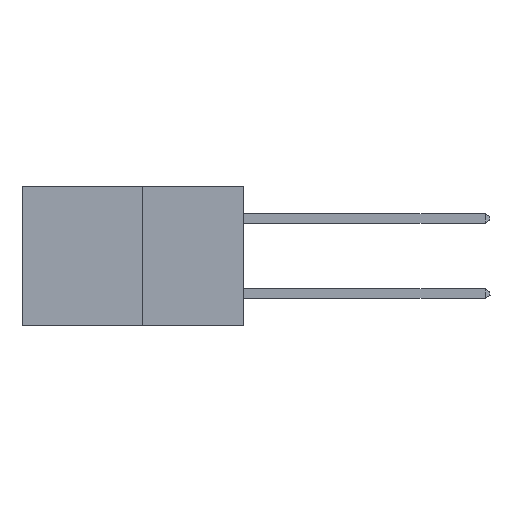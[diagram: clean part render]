
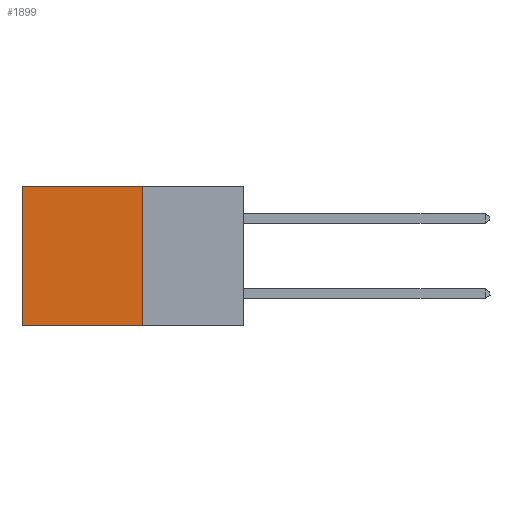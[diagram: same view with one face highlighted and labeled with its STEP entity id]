
A CAD part, left-side view. The second image highlights one B-rep face of the part: STEP entity #1899.
In plain terms, the highlighted planar face has unit normal (-1, 0, 0).
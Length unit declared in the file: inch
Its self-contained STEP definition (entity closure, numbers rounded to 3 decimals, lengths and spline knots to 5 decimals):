
#274 = EDGE_CURVE ( 'NONE', #8923, #3825, #8251, .T. ) ;
#282 = LINE ( 'NONE', #6244, #6192 ) ;
#631 = AXIS2_PLACEMENT_3D ( 'NONE', #7291, #9025, #3085 ) ;
#766 = EDGE_CURVE ( 'NONE', #3419, #8923, #282, .T. ) ;
#1061 = LINE ( 'NONE', #7419, #8402 ) ;
#1638 = ORIENTED_EDGE ( 'NONE', *, *, #3926, .T. ) ;
#1654 = ORIENTED_EDGE ( 'NONE', *, *, #274, .F. ) ;
#1670 = ORIENTED_EDGE ( 'NONE', *, *, #766, .F. ) ;
#1727 = ORIENTED_EDGE ( 'NONE', *, *, #7689, .T. ) ;
#1899 = ADVANCED_FACE ( 'NONE', ( #2489 ), #7920, .F. ) ;
#2247 = CARTESIAN_POINT ( 'NONE',  ( 0.277, 0.27, -0.37 ) ) ;
#2489 = FACE_OUTER_BOUND ( 'NONE', #4990, .T. ) ;
#2649 = CARTESIAN_POINT ( 'NONE',  ( 0.277, 0.59, -0.37 ) ) ;
#2954 = VERTEX_POINT ( 'NONE', #8623 ) ;
#3085 = DIRECTION ( 'NONE',  ( 0., 0., -1. ) ) ;
#3419 = VERTEX_POINT ( 'NONE', #3461 ) ;
#3461 = CARTESIAN_POINT ( 'NONE',  ( 0.277, 0.27, 0. ) ) ;
#3825 = VERTEX_POINT ( 'NONE', #2649 ) ;
#3926 = EDGE_CURVE ( 'NONE', #2954, #3825, #5712, .T. ) ;
#4722 = DIRECTION ( 'NONE',  ( 0., 0., -1. ) ) ;
#4990 = EDGE_LOOP ( 'NONE', ( #1638, #1654, #1670, #1727 ) ) ;
#5712 = LINE ( 'NONE', #7427, #7229 ) ;
#6192 = VECTOR ( 'NONE', #4722, 39.37008 ) ;
#6244 = CARTESIAN_POINT ( 'NONE',  ( 0.277, 0.27, -0.37 ) ) ;
#6470 = CARTESIAN_POINT ( 'NONE',  ( 0.277, 0.27, -0.37 ) ) ;
#7229 = VECTOR ( 'NONE', #8102, 39.37008 ) ;
#7291 = CARTESIAN_POINT ( 'NONE',  ( 0.277, 0.27, -0.37 ) ) ;
#7419 = CARTESIAN_POINT ( 'NONE',  ( 0.277, 0.27, 0. ) ) ;
#7427 = CARTESIAN_POINT ( 'NONE',  ( 0.277, 0.59, -0.37 ) ) ;
#7689 = EDGE_CURVE ( 'NONE', #3419, #2954, #1061, .T. ) ;
#7920 = PLANE ( 'NONE',  #631 ) ;
#8068 = VECTOR ( 'NONE', #8546, 39.37008 ) ;
#8095 = DIRECTION ( 'NONE',  ( 0., 1., 0. ) ) ;
#8102 = DIRECTION ( 'NONE',  ( 0., 0., -1. ) ) ;
#8251 = LINE ( 'NONE', #2247, #8068 ) ;
#8402 = VECTOR ( 'NONE', #8095, 39.37008 ) ;
#8546 = DIRECTION ( 'NONE',  ( 0., 1., 0. ) ) ;
#8623 = CARTESIAN_POINT ( 'NONE',  ( 0.277, 0.59, 0. ) ) ;
#8923 = VERTEX_POINT ( 'NONE', #6470 ) ;
#9025 = DIRECTION ( 'NONE',  ( 1., 0., 0. ) ) ;
